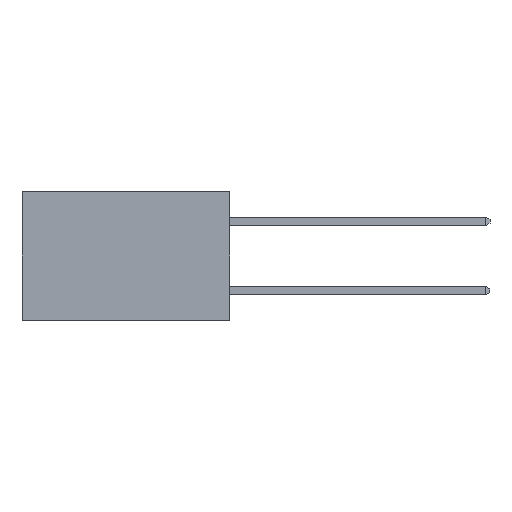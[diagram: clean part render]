
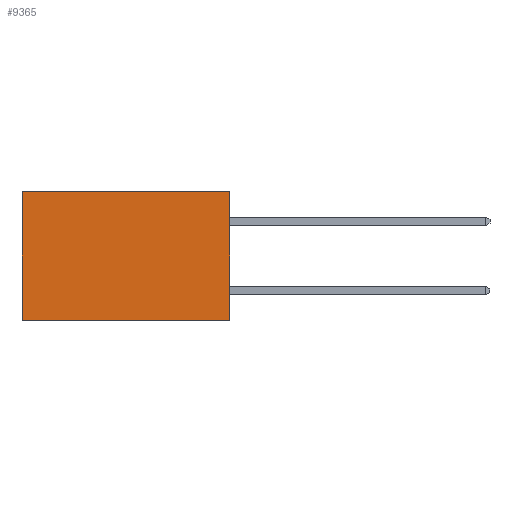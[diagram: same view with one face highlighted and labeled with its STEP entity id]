
A CAD part, left-side view. The second image highlights one B-rep face of the part: STEP entity #9365.
In plain terms, the highlighted planar face has unit normal (-1, 0, 0).
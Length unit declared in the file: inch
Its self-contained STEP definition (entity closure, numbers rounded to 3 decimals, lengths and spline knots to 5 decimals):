
#200 = CARTESIAN_POINT ( 'NONE',  ( 0.298, 0., 0. ) ) ;
#231 = DIRECTION ( 'NONE',  ( 0., 1., 0. ) ) ;
#515 = PLANE ( 'NONE',  #2220 ) ;
#1268 = LINE ( 'NONE', #5620, #11875 ) ;
#1888 = DIRECTION ( 'NONE',  ( 0., 0., -1. ) ) ;
#2220 = AXIS2_PLACEMENT_3D ( 'NONE', #5438, #9474, #3511 ) ;
#2370 = LINE ( 'NONE', #5147, #9976 ) ;
#2637 = CARTESIAN_POINT ( 'NONE',  ( 0.298, 0., -0.37 ) ) ;
#2683 = VERTEX_POINT ( 'NONE', #11616 ) ;
#2906 = ORIENTED_EDGE ( 'NONE', *, *, #8888, .T. ) ;
#3511 = DIRECTION ( 'NONE',  ( 0., 0., -1. ) ) ;
#3722 = VERTEX_POINT ( 'NONE', #7365 ) ;
#4268 = DIRECTION ( 'NONE',  ( 0., 1., 0. ) ) ;
#4739 = ORIENTED_EDGE ( 'NONE', *, *, #8595, .F. ) ;
#4855 = EDGE_CURVE ( 'NONE', #12265, #2683, #7117, .T. ) ;
#5147 = CARTESIAN_POINT ( 'NONE',  ( 0.298, 0., -0.37 ) ) ;
#5438 = CARTESIAN_POINT ( 'NONE',  ( 0.298, 0., 0. ) ) ;
#5620 = CARTESIAN_POINT ( 'NONE',  ( 0.298, 0.6, 0. ) ) ;
#7117 = LINE ( 'NONE', #200, #12168 ) ;
#7295 = CARTESIAN_POINT ( 'NONE',  ( 0.298, 0., 0. ) ) ;
#7365 = CARTESIAN_POINT ( 'NONE',  ( 0.298, 0.6, -0.37 ) ) ;
#8233 = ORIENTED_EDGE ( 'NONE', *, *, #9633, .F. ) ;
#8390 = VECTOR ( 'NONE', #1888, 39.37008 ) ;
#8595 = EDGE_CURVE ( 'NONE', #11085, #3722, #2370, .T. ) ;
#8848 = ORIENTED_EDGE ( 'NONE', *, *, #4855, .T. ) ;
#8878 = CARTESIAN_POINT ( 'NONE',  ( 0.298, 0., 0. ) ) ;
#8888 = EDGE_CURVE ( 'NONE', #2683, #3722, #1268, .T. ) ;
#9014 = LINE ( 'NONE', #8878, #8390 ) ;
#9178 = FACE_OUTER_BOUND ( 'NONE', #10245, .T. ) ;
#9365 = ADVANCED_FACE ( 'NONE', ( #9178 ), #515, .F. ) ;
#9474 = DIRECTION ( 'NONE',  ( 1., 0., 0. ) ) ;
#9633 = EDGE_CURVE ( 'NONE', #12265, #11085, #9014, .T. ) ;
#9976 = VECTOR ( 'NONE', #231, 39.37008 ) ;
#10245 = EDGE_LOOP ( 'NONE', ( #2906, #4739, #8233, #8848 ) ) ;
#11085 = VERTEX_POINT ( 'NONE', #2637 ) ;
#11616 = CARTESIAN_POINT ( 'NONE',  ( 0.298, 0.6, 0. ) ) ;
#11875 = VECTOR ( 'NONE', #12653, 39.37008 ) ;
#12168 = VECTOR ( 'NONE', #4268, 39.37008 ) ;
#12265 = VERTEX_POINT ( 'NONE', #7295 ) ;
#12653 = DIRECTION ( 'NONE',  ( 0., 0., -1. ) ) ;
